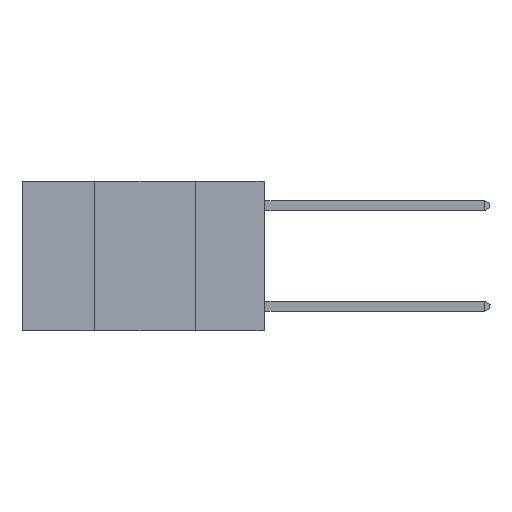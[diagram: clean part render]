
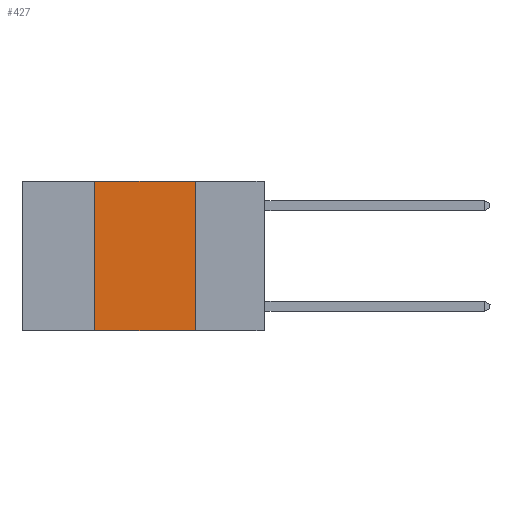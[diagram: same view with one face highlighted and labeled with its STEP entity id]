
A CAD part, left-side view. The second image highlights one B-rep face of the part: STEP entity #427.
In plain terms, the highlighted planar face has unit normal (-1, 0, 0).
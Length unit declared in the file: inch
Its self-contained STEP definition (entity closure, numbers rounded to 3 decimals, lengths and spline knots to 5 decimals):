
#427 = ADVANCED_FACE ( 'NONE', ( #10162 ), #3470, .F. ) ;
#1305 = CARTESIAN_POINT ( 'NONE',  ( 0., 0.6, 0. ) ) ;
#1350 = CARTESIAN_POINT ( 'NONE',  ( 0., 0.6, 0. ) ) ;
#1405 = VERTEX_POINT ( 'NONE', #4972 ) ;
#1484 = VECTOR ( 'NONE', #2189, 39.37008 ) ;
#1746 = ORIENTED_EDGE ( 'NONE', *, *, #9813, .T. ) ;
#1763 = LINE ( 'NONE', #8977, #1484 ) ;
#1906 = VECTOR ( 'NONE', #9724, 39.37008 ) ;
#2087 = VERTEX_POINT ( 'NONE', #6212 ) ;
#2189 = DIRECTION ( 'NONE',  ( 0., -1., 0. ) ) ;
#2298 = CARTESIAN_POINT ( 'NONE',  ( 0., 0.42, 0. ) ) ;
#2330 = CARTESIAN_POINT ( 'NONE',  ( 0., 0.17, 0. ) ) ;
#2525 = EDGE_CURVE ( 'NONE', #2087, #1405, #3989, .T. ) ;
#3151 = VERTEX_POINT ( 'NONE', #8397 ) ;
#3470 = PLANE ( 'NONE',  #6574 ) ;
#3823 = ORIENTED_EDGE ( 'NONE', *, *, #9827, .F. ) ;
#3972 = DIRECTION ( 'NONE',  ( 0., -1., 0. ) ) ;
#3989 = LINE ( 'NONE', #2330, #1906 ) ;
#4270 = DIRECTION ( 'NONE',  ( 0., 0., -1. ) ) ;
#4409 = VECTOR ( 'NONE', #8086, 39.37008 ) ;
#4972 = CARTESIAN_POINT ( 'NONE',  ( 0., 0.17, -0.37 ) ) ;
#5802 = LINE ( 'NONE', #1350, #10235 ) ;
#6212 = CARTESIAN_POINT ( 'NONE',  ( 0., 0.17, 0. ) ) ;
#6574 = AXIS2_PLACEMENT_3D ( 'NONE', #1305, #10726, #4270 ) ;
#6575 = ORIENTED_EDGE ( 'NONE', *, *, #8292, .F. ) ;
#7263 = CARTESIAN_POINT ( 'NONE',  ( 0., 0.42, 0. ) ) ;
#8086 = DIRECTION ( 'NONE',  ( 0., 0., 1. ) ) ;
#8292 = EDGE_CURVE ( 'NONE', #3151, #9878, #8844, .T. ) ;
#8397 = CARTESIAN_POINT ( 'NONE',  ( 0., 0.42, -0.37 ) ) ;
#8678 = EDGE_LOOP ( 'NONE', ( #10486, #3823, #6575, #1746 ) ) ;
#8844 = LINE ( 'NONE', #7263, #4409 ) ;
#8977 = CARTESIAN_POINT ( 'NONE',  ( 0., 0.6, -0.37 ) ) ;
#9724 = DIRECTION ( 'NONE',  ( 0., 0., -1. ) ) ;
#9813 = EDGE_CURVE ( 'NONE', #3151, #1405, #1763, .T. ) ;
#9827 = EDGE_CURVE ( 'NONE', #9878, #2087, #5802, .T. ) ;
#9878 = VERTEX_POINT ( 'NONE', #2298 ) ;
#10162 = FACE_OUTER_BOUND ( 'NONE', #8678, .T. ) ;
#10235 = VECTOR ( 'NONE', #3972, 39.37008 ) ;
#10486 = ORIENTED_EDGE ( 'NONE', *, *, #2525, .F. ) ;
#10726 = DIRECTION ( 'NONE',  ( 1., 0., 0. ) ) ;
